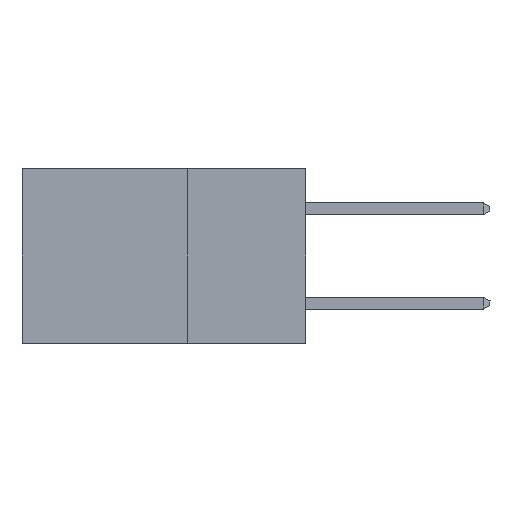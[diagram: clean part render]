
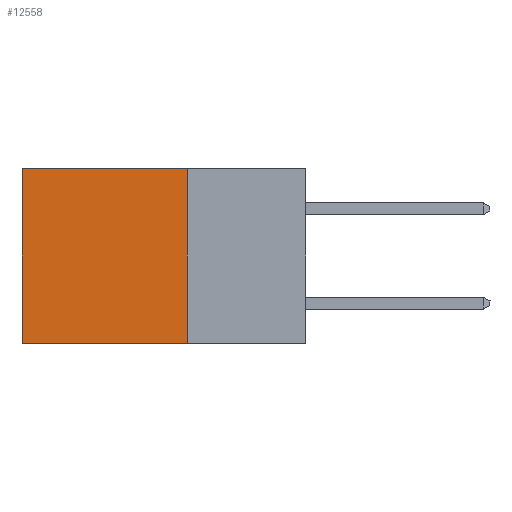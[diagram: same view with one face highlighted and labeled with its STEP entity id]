
A CAD part, left-side view. The second image highlights one B-rep face of the part: STEP entity #12558.
In plain terms, the highlighted planar face has unit normal (-1, 0, 0).
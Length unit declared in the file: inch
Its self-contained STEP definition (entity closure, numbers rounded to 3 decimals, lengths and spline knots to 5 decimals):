
#211 = VECTOR ( 'NONE', #2214, 39.37008 ) ;
#1019 = ORIENTED_EDGE ( 'NONE', *, *, #1391, .F. ) ;
#1391 = EDGE_CURVE ( 'NONE', #10851, #3919, #7996, .T. ) ;
#2214 = DIRECTION ( 'NONE',  ( 0., 1., 0. ) ) ;
#2515 = DIRECTION ( 'NONE',  ( 0., 0., -1. ) ) ;
#2623 = LINE ( 'NONE', #13089, #12018 ) ;
#2962 = CARTESIAN_POINT ( 'NONE',  ( 0.298, 0.6, -0.37 ) ) ;
#3114 = CARTESIAN_POINT ( 'NONE',  ( 0.298, 0.25, -0.37 ) ) ;
#3887 = CARTESIAN_POINT ( 'NONE',  ( 0.298, 0.25, -0.37 ) ) ;
#3919 = VERTEX_POINT ( 'NONE', #3114 ) ;
#3979 = CARTESIAN_POINT ( 'NONE',  ( 0.298, 0.25, 0. ) ) ;
#4039 = EDGE_CURVE ( 'NONE', #10851, #9378, #6095, .T. ) ;
#4148 = DIRECTION ( 'NONE',  ( 0., 0., -1. ) ) ;
#4632 = AXIS2_PLACEMENT_3D ( 'NONE', #3979, #10295, #2515 ) ;
#4745 = EDGE_CURVE ( 'NONE', #9378, #5980, #2623, .T. ) ;
#4921 = LINE ( 'NONE', #3887, #6801 ) ;
#5980 = VERTEX_POINT ( 'NONE', #2962 ) ;
#6095 = LINE ( 'NONE', #13352, #211 ) ;
#6363 = ORIENTED_EDGE ( 'NONE', *, *, #4039, .T. ) ;
#6510 = CARTESIAN_POINT ( 'NONE',  ( 0.298, 0.25, 0. ) ) ;
#6646 = DIRECTION ( 'NONE',  ( 0., 0., -1. ) ) ;
#6690 = CARTESIAN_POINT ( 'NONE',  ( 0.298, 0.6, 0. ) ) ;
#6801 = VECTOR ( 'NONE', #8178, 39.37008 ) ;
#6947 = VECTOR ( 'NONE', #6646, 39.37008 ) ;
#7996 = LINE ( 'NONE', #6510, #6947 ) ;
#8178 = DIRECTION ( 'NONE',  ( 0., 1., 0. ) ) ;
#8525 = ORIENTED_EDGE ( 'NONE', *, *, #4745, .T. ) ;
#8911 = FACE_OUTER_BOUND ( 'NONE', #13305, .T. ) ;
#9378 = VERTEX_POINT ( 'NONE', #6690 ) ;
#9798 = CARTESIAN_POINT ( 'NONE',  ( 0.298, 0.25, 0. ) ) ;
#10014 = ORIENTED_EDGE ( 'NONE', *, *, #12418, .F. ) ;
#10295 = DIRECTION ( 'NONE',  ( 1., 0., 0. ) ) ;
#10851 = VERTEX_POINT ( 'NONE', #9798 ) ;
#12018 = VECTOR ( 'NONE', #4148, 39.37008 ) ;
#12418 = EDGE_CURVE ( 'NONE', #3919, #5980, #4921, .T. ) ;
#12558 = ADVANCED_FACE ( 'NONE', ( #8911 ), #12861, .F. ) ;
#12861 = PLANE ( 'NONE',  #4632 ) ;
#13089 = CARTESIAN_POINT ( 'NONE',  ( 0.298, 0.6, 0. ) ) ;
#13305 = EDGE_LOOP ( 'NONE', ( #8525, #10014, #1019, #6363 ) ) ;
#13352 = CARTESIAN_POINT ( 'NONE',  ( 0.298, 0.25, 0. ) ) ;
